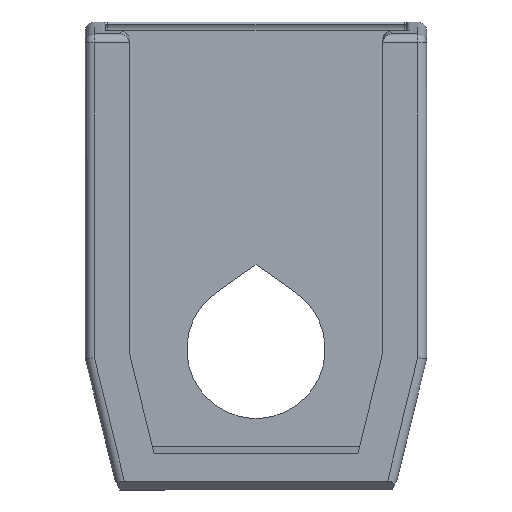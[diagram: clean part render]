
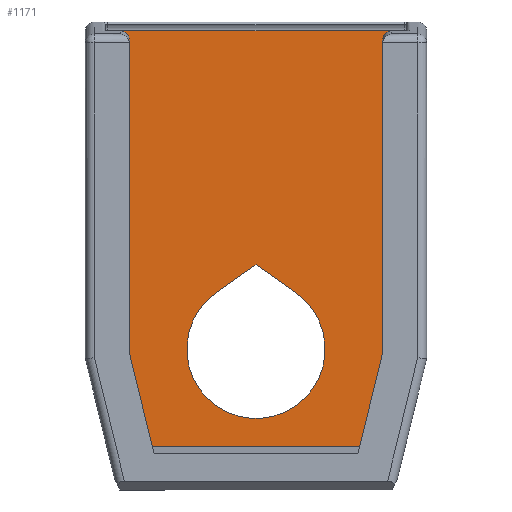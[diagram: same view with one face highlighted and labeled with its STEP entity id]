
A CAD part, front view. The second image highlights one B-rep face of the part: STEP entity #1171.
In plain terms, the highlighted planar face has unit normal (0, 1, 0).
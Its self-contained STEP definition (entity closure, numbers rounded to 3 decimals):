
#15=FACE_BOUND('',#207,.T.);
#53=CIRCLE('',#1308,5.8);
#137=FACE_OUTER_BOUND('',#206,.T.);
#206=EDGE_LOOP('',(#966,#967,#968,#969,#970,#971,#972,#973));
#207=EDGE_LOOP('',(#974,#975,#976));
#307=LINE('',#1908,#417);
#310=LINE('',#1923,#420);
#312=LINE('',#1928,#422);
#314=LINE('',#1942,#424);
#315=LINE('',#1944,#425);
#317=LINE('',#1949,#427);
#328=LINE('',#2009,#438);
#335=LINE('',#2034,#445);
#336=LINE('',#2037,#446);
#337=LINE('',#2040,#447);
#417=VECTOR('',#1475,10.);
#420=VECTOR('',#1496,10.);
#422=VECTOR('',#1502,10.);
#424=VECTOR('',#1520,10.);
#425=VECTOR('',#1523,10.);
#427=VECTOR('',#1527,10.);
#438=VECTOR('',#1582,10.);
#445=VECTOR('',#1613,10.);
#446=VECTOR('',#1614,10.);
#447=VECTOR('',#1617,10.);
#535=VERTEX_POINT('',#1905);
#536=VERTEX_POINT('',#1907);
#539=VERTEX_POINT('',#1919);
#540=VERTEX_POINT('',#1926);
#543=VERTEX_POINT('',#1936);
#544=VERTEX_POINT('',#1940);
#546=VERTEX_POINT('',#1948);
#558=VERTEX_POINT('',#2008);
#565=VERTEX_POINT('',#2035);
#566=VERTEX_POINT('',#2036);
#567=VERTEX_POINT('',#2038);
#660=EDGE_CURVE('',#535,#536,#307,.T.);
#668=EDGE_CURVE('',#536,#539,#310,.T.);
#671=EDGE_CURVE('',#539,#540,#312,.T.);
#678=EDGE_CURVE('',#544,#543,#314,.T.);
#679=EDGE_CURVE('',#540,#544,#315,.T.);
#681=EDGE_CURVE('',#543,#546,#317,.T.);
#705=EDGE_CURVE('',#546,#558,#328,.T.);
#718=EDGE_CURVE('',#558,#535,#335,.T.);
#719=EDGE_CURVE('',#565,#566,#336,.T.);
#720=EDGE_CURVE('',#567,#565,#53,.T.);
#721=EDGE_CURVE('',#566,#567,#337,.T.);
#966=ORIENTED_EDGE('',*,*,#705,.F.);
#967=ORIENTED_EDGE('',*,*,#681,.F.);
#968=ORIENTED_EDGE('',*,*,#678,.F.);
#969=ORIENTED_EDGE('',*,*,#679,.F.);
#970=ORIENTED_EDGE('',*,*,#671,.F.);
#971=ORIENTED_EDGE('',*,*,#668,.F.);
#972=ORIENTED_EDGE('',*,*,#660,.F.);
#973=ORIENTED_EDGE('',*,*,#718,.F.);
#974=ORIENTED_EDGE('',*,*,#719,.F.);
#975=ORIENTED_EDGE('',*,*,#720,.F.);
#976=ORIENTED_EDGE('',*,*,#721,.F.);
#1104=PLANE('',#1307);
#1171=ADVANCED_FACE('',(#137,#15),#1104,.F.);
#1307=AXIS2_PLACEMENT_3D('',#2033,#1611,#1612);
#1308=AXIS2_PLACEMENT_3D('',#2039,#1615,#1616);
#1475=DIRECTION('',(0.237,0.,0.971));
#1496=DIRECTION('',(0.,0.,1.));
#1502=DIRECTION('',(-1.,0.,0.));
#1520=DIRECTION('',(-1.,0.,0.));
#1523=DIRECTION('',(-1.,0.,0.));
#1527=DIRECTION('',(0.,0.,-1.));
#1582=DIRECTION('',(0.237,0.,-0.971));
#1611=DIRECTION('center_axis',(0.,-1.,0.));
#1612=DIRECTION('ref_axis',(1.,0.,0.));
#1613=DIRECTION('',(1.,0.,0.));
#1614=DIRECTION('',(0.819,0.,0.574));
#1615=DIRECTION('center_axis',(0.,1.,0.));
#1616=DIRECTION('ref_axis',(-0.574,0.,0.819));
#1617=DIRECTION('',(0.819,0.,-0.574));
#1905=CARTESIAN_POINT('',(11.028,-15.675,0.75));
#1907=CARTESIAN_POINT('',(13.55,-15.675,11.083));
#1908=CARTESIAN_POINT('',(12.797,-15.675,8.));
#1919=CARTESIAN_POINT('',(13.55,-15.675,38.473));
#1923=CARTESIAN_POINT('',(13.55,-15.675,15.202));
#1926=CARTESIAN_POINT('',(12.434,-15.675,38.473));
#1928=CARTESIAN_POINT('',(7.15,-15.675,38.473));
#1936=CARTESIAN_POINT('',(-13.55,-15.675,38.473));
#1940=CARTESIAN_POINT('',(-12.434,-15.675,38.473));
#1942=CARTESIAN_POINT('',(-6.217,-15.675,38.473));
#1944=CARTESIAN_POINT('',(6.217,-15.675,38.473));
#1948=CARTESIAN_POINT('',(-13.55,-15.675,11.083));
#1949=CARTESIAN_POINT('',(-13.55,-15.675,29.118));
#2008=CARTESIAN_POINT('',(-11.028,-15.675,0.75));
#2009=CARTESIAN_POINT('',(-14.139,-15.675,13.496));
#2033=CARTESIAN_POINT('Origin',(0.,-15.675,19.412));
#2034=CARTESIAN_POINT('',(-5.808,-15.675,0.75));
#2035=CARTESIAN_POINT('',(-3.327,-15.675,16.551));
#2036=CARTESIAN_POINT('',(0.,-15.675,18.88));
#2037=CARTESIAN_POINT('',(0.,-15.675,18.88));
#2038=CARTESIAN_POINT('',(3.327,-15.675,16.551));
#2039=CARTESIAN_POINT('Origin',(0.,-15.675,11.8));
#2040=CARTESIAN_POINT('',(0.,-15.675,18.88));
